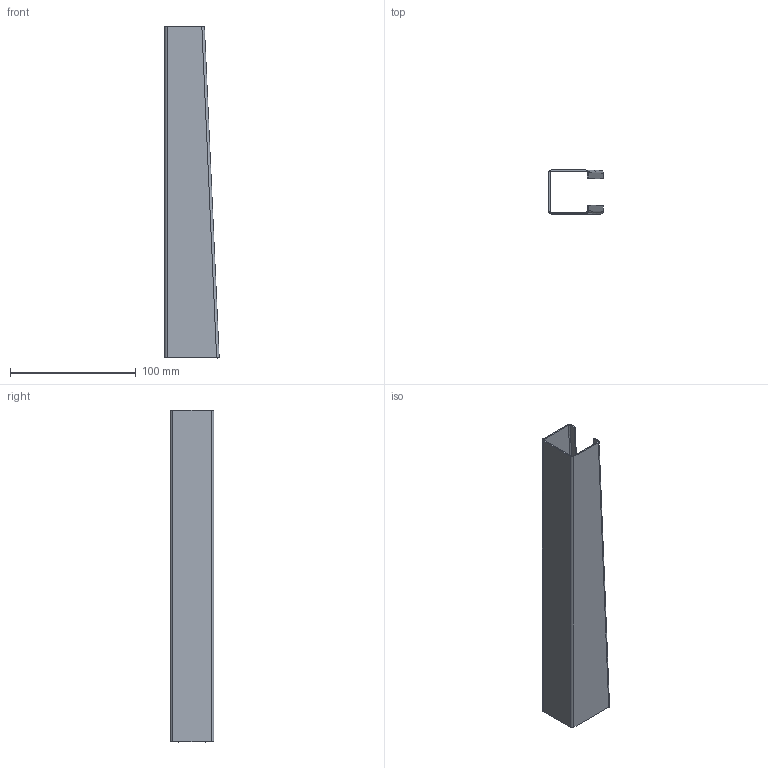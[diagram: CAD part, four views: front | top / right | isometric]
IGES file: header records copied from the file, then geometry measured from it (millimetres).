
Start section: SolidWorks IGES FILE using analytic representation for surfaces
Global section: file name: AK47_Blank.IGS; native system: SolidWorks 2004 by SolidWorks Corporation; preprocessor: Version 5.3; author: Me; date: 040229.194007; units: inch
Bounding box: 43.18 x 34.53 x 263.8 mm (x, y, z)
Surface area: 61690.5 mm2 (no closed solid volume)
Topology: 0 solids, 0 shells, 38 faces, 208 edges, 208 vertices
Faces by surface type: bspline 30, revolution 8
